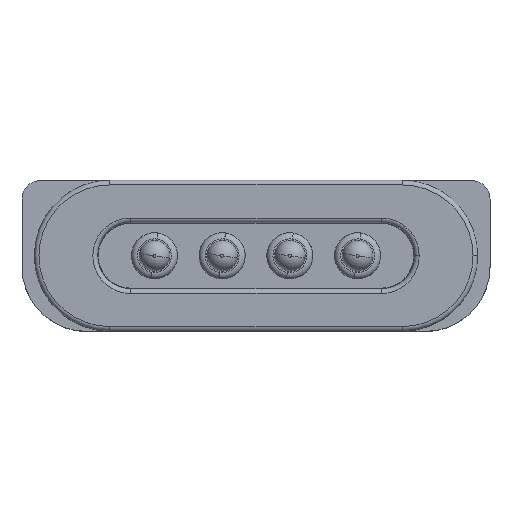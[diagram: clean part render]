
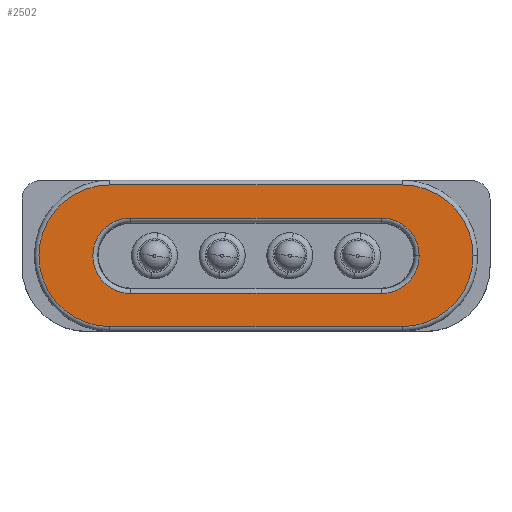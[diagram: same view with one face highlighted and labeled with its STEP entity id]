
A CAD part, top view. The second image highlights one B-rep face of the part: STEP entity #2502.
In plain terms, the highlighted planar face has unit normal (0, 0, 1).
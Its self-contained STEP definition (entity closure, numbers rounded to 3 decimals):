
#82 = DIRECTION ( 'NONE',  ( -1., 0., 0. ) ) ;
#501 = CIRCLE ( 'NONE', #6887, 1.225 ) ;
#524 = VERTEX_POINT ( 'NONE', #2520 ) ;
#609 = CARTESIAN_POINT ( 'NONE',  ( 4.75, 50., 2. ) ) ;
#671 = CARTESIAN_POINT ( 'NONE',  ( 4.75, 52.3, 2. ) ) ;
#748 = DIRECTION ( 'NONE',  ( 0., 0., -1. ) ) ;
#810 = CARTESIAN_POINT ( 'NONE',  ( -4.075, 50., 2. ) ) ;
#983 = CIRCLE ( 'NONE', #8857, 2.3 ) ;
#1079 = EDGE_CURVE ( 'NONE', #524, #6414, #4754, .T. ) ;
#1131 = DIRECTION ( 'NONE',  ( 1., 0., 0. ) ) ;
#1227 = EDGE_LOOP ( 'NONE', ( #8891, #5010, #3945, #1527, #8149 ) ) ;
#1272 = EDGE_CURVE ( 'NONE', #6570, #7491, #1368, .T. ) ;
#1343 = DIRECTION ( 'NONE',  ( -1., 0., 0. ) ) ;
#1368 = CIRCLE ( 'NONE', #1797, 2.3 ) ;
#1406 = CARTESIAN_POINT ( 'NONE',  ( 4.075, 50., 2. ) ) ;
#1527 = ORIENTED_EDGE ( 'NONE', *, *, #7674, .T. ) ;
#1682 = CARTESIAN_POINT ( 'NONE',  ( 4.075, 51.225, 2. ) ) ;
#1701 = CIRCLE ( 'NONE', #8519, 2.3 ) ;
#1732 = ORIENTED_EDGE ( 'NONE', *, *, #1079, .T. ) ;
#1754 = DIRECTION ( 'NONE',  ( -1., 0., 0. ) ) ;
#1797 = AXIS2_PLACEMENT_3D ( 'NONE', #7718, #4212, #1343 ) ;
#2120 = DIRECTION ( 'NONE',  ( 0., 0., 1. ) ) ;
#2148 = EDGE_CURVE ( 'NONE', #5528, #2886, #501, .T. ) ;
#2502 = ADVANCED_FACE ( 'NONE', ( #5903, #5995 ), #8137, .T. ) ;
#2520 = CARTESIAN_POINT ( 'NONE',  ( 5.3, 50., 2. ) ) ;
#2636 = DIRECTION ( 'NONE',  ( 0., -1., 0. ) ) ;
#2681 = VECTOR ( 'NONE', #1754, 1000. ) ;
#2714 = DIRECTION ( 'NONE',  ( 0., 0., 1. ) ) ;
#2827 = LINE ( 'NONE', #9169, #4681 ) ;
#2886 = VERTEX_POINT ( 'NONE', #7624 ) ;
#3523 = CARTESIAN_POINT ( 'NONE',  ( 4.075, 50., 2. ) ) ;
#3945 = ORIENTED_EDGE ( 'NONE', *, *, #4370, .T. ) ;
#4003 = AXIS2_PLACEMENT_3D ( 'NONE', #8320, #2714, #7731 ) ;
#4191 = ORIENTED_EDGE ( 'NONE', *, *, #6018, .T. ) ;
#4205 = ORIENTED_EDGE ( 'NONE', *, *, #5461, .T. ) ;
#4212 = DIRECTION ( 'NONE',  ( 0., 0., 1. ) ) ;
#4244 = VERTEX_POINT ( 'NONE', #6906 ) ;
#4273 = VECTOR ( 'NONE', #1131, 1000. ) ;
#4370 = EDGE_CURVE ( 'NONE', #7491, #4244, #2827, .T. ) ;
#4400 = LINE ( 'NONE', #6636, #2681 ) ;
#4681 = VECTOR ( 'NONE', #7830, 1000. ) ;
#4754 = CIRCLE ( 'NONE', #8324, 1.225 ) ;
#4869 = DIRECTION ( 'NONE',  ( 0., 1., 0. ) ) ;
#5010 = ORIENTED_EDGE ( 'NONE', *, *, #1272, .T. ) ;
#5310 = CARTESIAN_POINT ( 'NONE',  ( 4.075, 48.775, 2. ) ) ;
#5461 = EDGE_CURVE ( 'NONE', #2886, #5479, #6082, .T. ) ;
#5478 = CARTESIAN_POINT ( 'NONE',  ( -4.075, 48.775, 2. ) ) ;
#5479 = VERTEX_POINT ( 'NONE', #1682 ) ;
#5528 = VERTEX_POINT ( 'NONE', #5478 ) ;
#5595 = ORIENTED_EDGE ( 'NONE', *, *, #5615, .T. ) ;
#5615 = EDGE_CURVE ( 'NONE', #5479, #524, #8797, .T. ) ;
#5773 = DIRECTION ( 'NONE',  ( 0., -1., 0. ) ) ;
#5903 = FACE_BOUND ( 'NONE', #6573, .T. ) ;
#5995 = FACE_OUTER_BOUND ( 'NONE', #1227, .T. ) ;
#6018 = EDGE_CURVE ( 'NONE', #6414, #5528, #4400, .T. ) ;
#6082 = LINE ( 'NONE', #8935, #4273 ) ;
#6307 = DIRECTION ( 'NONE',  ( 0., 0., -1. ) ) ;
#6320 = CARTESIAN_POINT ( 'NONE',  ( 4.75, 50., 2. ) ) ;
#6405 = AXIS2_PLACEMENT_3D ( 'NONE', #1406, #748, #8551 ) ;
#6414 = VERTEX_POINT ( 'NONE', #5310 ) ;
#6416 = CARTESIAN_POINT ( 'NONE',  ( 7.05, 50., 2. ) ) ;
#6467 = DIRECTION ( 'NONE',  ( 0., 0., -1. ) ) ;
#6542 = LINE ( 'NONE', #8646, #8861 ) ;
#6549 = CARTESIAN_POINT ( 'NONE',  ( -4.75, 52.3, 2. ) ) ;
#6570 = VERTEX_POINT ( 'NONE', #6549 ) ;
#6573 = EDGE_LOOP ( 'NONE', ( #5595, #1732, #4191, #7083, #4205 ) ) ;
#6636 = CARTESIAN_POINT ( 'NONE',  ( 4.075, 48.775, 2. ) ) ;
#6846 = DIRECTION ( 'NONE',  ( 0., 0., 1. ) ) ;
#6887 = AXIS2_PLACEMENT_3D ( 'NONE', #810, #6467, #5773 ) ;
#6906 = CARTESIAN_POINT ( 'NONE',  ( 4.75, 47.7, 2. ) ) ;
#7064 = EDGE_CURVE ( 'NONE', #8672, #9202, #1701, .T. ) ;
#7083 = ORIENTED_EDGE ( 'NONE', *, *, #2148, .T. ) ;
#7491 = VERTEX_POINT ( 'NONE', #8438 ) ;
#7624 = CARTESIAN_POINT ( 'NONE',  ( -4.075, 51.225, 2. ) ) ;
#7674 = EDGE_CURVE ( 'NONE', #4244, #8672, #983, .T. ) ;
#7718 = CARTESIAN_POINT ( 'NONE',  ( -4.75, 50., 2. ) ) ;
#7731 = DIRECTION ( 'NONE',  ( 1., 0., 0. ) ) ;
#7752 = EDGE_CURVE ( 'NONE', #9202, #6570, #6542, .T. ) ;
#7830 = DIRECTION ( 'NONE',  ( 1., 0., 0. ) ) ;
#8137 = PLANE ( 'NONE',  #4003 ) ;
#8149 = ORIENTED_EDGE ( 'NONE', *, *, #7064, .T. ) ;
#8320 = CARTESIAN_POINT ( 'NONE',  ( 0.001, 50., 2. ) ) ;
#8324 = AXIS2_PLACEMENT_3D ( 'NONE', #3523, #6307, #4869 ) ;
#8438 = CARTESIAN_POINT ( 'NONE',  ( -4.75, 47.7, 2. ) ) ;
#8459 = DIRECTION ( 'NONE',  ( 0., -1., 0. ) ) ;
#8519 = AXIS2_PLACEMENT_3D ( 'NONE', #6320, #6846, #2636 ) ;
#8551 = DIRECTION ( 'NONE',  ( 0., 1., 0. ) ) ;
#8646 = CARTESIAN_POINT ( 'NONE',  ( 4.75, 52.3, 2. ) ) ;
#8672 = VERTEX_POINT ( 'NONE', #6416 ) ;
#8797 = CIRCLE ( 'NONE', #6405, 1.225 ) ;
#8857 = AXIS2_PLACEMENT_3D ( 'NONE', #609, #2120, #8459 ) ;
#8861 = VECTOR ( 'NONE', #82, 1000. ) ;
#8891 = ORIENTED_EDGE ( 'NONE', *, *, #7752, .T. ) ;
#8935 = CARTESIAN_POINT ( 'NONE',  ( -4.075, 51.225, 2. ) ) ;
#9169 = CARTESIAN_POINT ( 'NONE',  ( -4.75, 47.7, 2. ) ) ;
#9202 = VERTEX_POINT ( 'NONE', #671 ) ;
